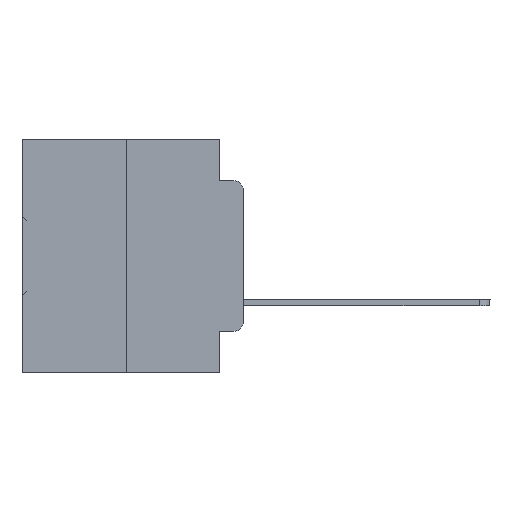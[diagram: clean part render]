
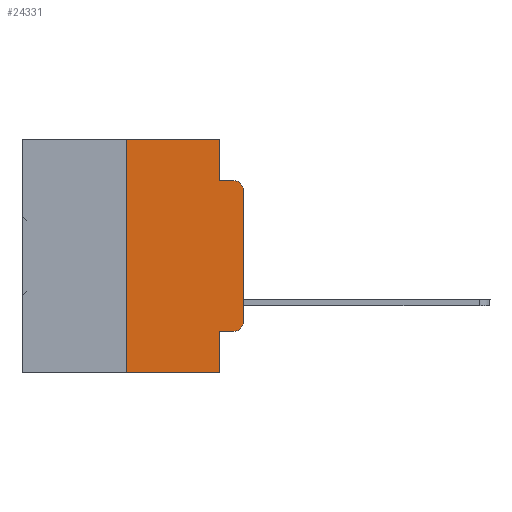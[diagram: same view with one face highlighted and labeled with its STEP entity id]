
A CAD part, left-side view. The second image highlights one B-rep face of the part: STEP entity #24331.
In plain terms, the highlighted planar face has unit normal (-1, 0, 0).
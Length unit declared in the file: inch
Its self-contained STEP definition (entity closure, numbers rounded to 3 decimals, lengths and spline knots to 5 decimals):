
#199 = VERTEX_POINT ( 'NONE', #37883 ) ;
#522 = DIRECTION ( 'NONE',  ( 0., -1., 0. ) ) ;
#1170 = VERTEX_POINT ( 'NONE', #32984 ) ;
#2089 = LINE ( 'NONE', #33539, #33260 ) ;
#2110 = CARTESIAN_POINT ( 'NONE',  ( 0., 0.25, 0. ) ) ;
#2490 = EDGE_CURVE ( 'NONE', #1170, #27609, #15487, .T. ) ;
#3181 = EDGE_LOOP ( 'NONE', ( #15927, #4767, #31269, #7522, #37802, #8353, #5724, #20904, #7162, #10452 ) ) ;
#3221 = CARTESIAN_POINT ( 'NONE',  ( 0., 0.051, -0.4115 ) ) ;
#3345 = EDGE_CURVE ( 'NONE', #5688, #16630, #8969, .T. ) ;
#3438 = EDGE_CURVE ( 'NONE', #11362, #29635, #33593, .T. ) ;
#3766 = CARTESIAN_POINT ( 'NONE',  ( 0., 0.473, 0. ) ) ;
#4509 = FACE_OUTER_BOUND ( 'NONE', #3181, .T. ) ;
#4767 = ORIENTED_EDGE ( 'NONE', *, *, #3345, .T. ) ;
#5289 = CARTESIAN_POINT ( 'NONE',  ( 0., 0.02, -0.4115 ) ) ;
#5401 = VERTEX_POINT ( 'NONE', #2110 ) ;
#5682 = EDGE_CURVE ( 'NONE', #11362, #5401, #24308, .T. ) ;
#5688 = VERTEX_POINT ( 'NONE', #30262 ) ;
#5724 = ORIENTED_EDGE ( 'NONE', *, *, #3438, .T. ) ;
#5741 = CARTESIAN_POINT ( 'NONE',  ( 0., 0.051, -0.0885 ) ) ;
#5803 = DIRECTION ( 'NONE',  ( 0., 0., -1. ) ) ;
#5962 = EDGE_CURVE ( 'NONE', #5401, #21053, #35389, .T. ) ;
#7162 = ORIENTED_EDGE ( 'NONE', *, *, #2490, .T. ) ;
#7291 = DIRECTION ( 'NONE',  ( 0., 0., 1. ) ) ;
#7330 = CARTESIAN_POINT ( 'NONE',  ( 0., 0.02, -0.3915 ) ) ;
#7522 = ORIENTED_EDGE ( 'NONE', *, *, #26879, .F. ) ;
#8353 = ORIENTED_EDGE ( 'NONE', *, *, #5682, .F. ) ;
#8429 = DIRECTION ( 'NONE',  ( 0., 0., -1. ) ) ;
#8897 = AXIS2_PLACEMENT_3D ( 'NONE', #3766, #36142, #24817 ) ;
#8969 = CIRCLE ( 'NONE', #31617, 0.02 ) ;
#9660 = CARTESIAN_POINT ( 'NONE',  ( 0., 0.473, -0.5 ) ) ;
#10452 = ORIENTED_EDGE ( 'NONE', *, *, #20747, .T. ) ;
#10792 = CARTESIAN_POINT ( 'NONE',  ( 0., 0.051, -0.5 ) ) ;
#11108 = CARTESIAN_POINT ( 'NONE',  ( 0., 0.02, -0.0885 ) ) ;
#11354 = VECTOR ( 'NONE', #19030, 39.37008 ) ;
#11362 = VERTEX_POINT ( 'NONE', #21401 ) ;
#12023 = CARTESIAN_POINT ( 'NONE',  ( 0., 0.473, 0. ) ) ;
#12280 = CARTESIAN_POINT ( 'NONE',  ( 0., 0.051, 0. ) ) ;
#12959 = VECTOR ( 'NONE', #8429, 39.37008 ) ;
#15120 = VERTEX_POINT ( 'NONE', #18773 ) ;
#15487 = LINE ( 'NONE', #3221, #15718 ) ;
#15718 = VECTOR ( 'NONE', #522, 39.37008 ) ;
#15927 = ORIENTED_EDGE ( 'NONE', *, *, #21247, .T. ) ;
#16521 = DIRECTION ( 'NONE',  ( 0., 0., -1. ) ) ;
#16630 = VERTEX_POINT ( 'NONE', #11108 ) ;
#17866 = EDGE_CURVE ( 'NONE', #1170, #29635, #23158, .T. ) ;
#18079 = DIRECTION ( 'NONE',  ( -1., 0., 0. ) ) ;
#18773 = CARTESIAN_POINT ( 'NONE',  ( 0., 0., -0.3915 ) ) ;
#19030 = DIRECTION ( 'NONE',  ( 0., -1., 0. ) ) ;
#19255 = VECTOR ( 'NONE', #24501, 39.37008 ) ;
#20483 = LINE ( 'NONE', #5741, #30928 ) ;
#20570 = CARTESIAN_POINT ( 'NONE',  ( 0., 0.02, -0.1085 ) ) ;
#20747 = EDGE_CURVE ( 'NONE', #27609, #15120, #24064, .T. ) ;
#20904 = ORIENTED_EDGE ( 'NONE', *, *, #17866, .F. ) ;
#21053 = VERTEX_POINT ( 'NONE', #12280 ) ;
#21247 = EDGE_CURVE ( 'NONE', #15120, #5688, #2089, .T. ) ;
#21401 = CARTESIAN_POINT ( 'NONE',  ( 0., 0.25, -0.5 ) ) ;
#22077 = DIRECTION ( 'NONE',  ( -1., 0., 0. ) ) ;
#22355 = VECTOR ( 'NONE', #29074, 39.37008 ) ;
#23158 = LINE ( 'NONE', #34845, #12959 ) ;
#24064 = CIRCLE ( 'NONE', #34471, 0.02 ) ;
#24187 = EDGE_CURVE ( 'NONE', #199, #16630, #20483, .T. ) ;
#24308 = LINE ( 'NONE', #27186, #19255 ) ;
#24331 = ADVANCED_FACE ( 'NONE', ( #4509 ), #35764, .F. ) ;
#24501 = DIRECTION ( 'NONE',  ( 0., 0., 1. ) ) ;
#24817 = DIRECTION ( 'NONE',  ( 0., 0., -1. ) ) ;
#26879 = EDGE_CURVE ( 'NONE', #21053, #199, #32058, .T. ) ;
#27186 = CARTESIAN_POINT ( 'NONE',  ( 0., 0.25, 0. ) ) ;
#27609 = VERTEX_POINT ( 'NONE', #5289 ) ;
#29074 = DIRECTION ( 'NONE',  ( 0., -1., 0. ) ) ;
#29635 = VERTEX_POINT ( 'NONE', #10792 ) ;
#29774 = DIRECTION ( 'NONE',  ( 0., 0., -1. ) ) ;
#30262 = CARTESIAN_POINT ( 'NONE',  ( 0., 0., -0.1085 ) ) ;
#30469 = VECTOR ( 'NONE', #5803, 39.37008 ) ;
#30928 = VECTOR ( 'NONE', #32690, 39.37008 ) ;
#31269 = ORIENTED_EDGE ( 'NONE', *, *, #24187, .F. ) ;
#31617 = AXIS2_PLACEMENT_3D ( 'NONE', #20570, #18079, #29774 ) ;
#32058 = LINE ( 'NONE', #33330, #30469 ) ;
#32690 = DIRECTION ( 'NONE',  ( 0., -1., 0. ) ) ;
#32984 = CARTESIAN_POINT ( 'NONE',  ( 0., 0.051, -0.4115 ) ) ;
#33260 = VECTOR ( 'NONE', #7291, 39.37008 ) ;
#33330 = CARTESIAN_POINT ( 'NONE',  ( 0., 0.051, 0. ) ) ;
#33539 = CARTESIAN_POINT ( 'NONE',  ( 0., 0., 0. ) ) ;
#33593 = LINE ( 'NONE', #9660, #11354 ) ;
#34471 = AXIS2_PLACEMENT_3D ( 'NONE', #7330, #22077, #16521 ) ;
#34845 = CARTESIAN_POINT ( 'NONE',  ( 0., 0.051, 0. ) ) ;
#35389 = LINE ( 'NONE', #12023, #22355 ) ;
#35764 = PLANE ( 'NONE',  #8897 ) ;
#36142 = DIRECTION ( 'NONE',  ( 1., 0., 0. ) ) ;
#37802 = ORIENTED_EDGE ( 'NONE', *, *, #5962, .F. ) ;
#37883 = CARTESIAN_POINT ( 'NONE',  ( 0., 0.051, -0.0885 ) ) ;
